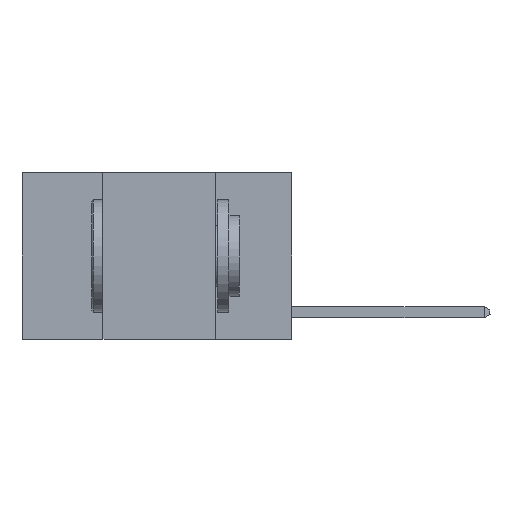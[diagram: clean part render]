
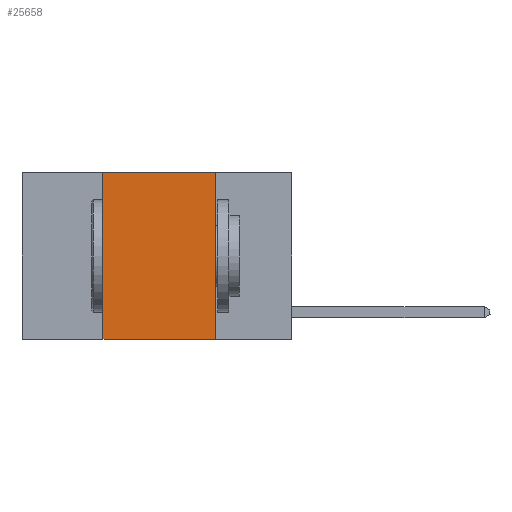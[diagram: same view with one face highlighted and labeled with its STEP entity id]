
A CAD part, left-side view. The second image highlights one B-rep face of the part: STEP entity #25658.
In plain terms, the highlighted planar face has unit normal (-1, 0, 0).
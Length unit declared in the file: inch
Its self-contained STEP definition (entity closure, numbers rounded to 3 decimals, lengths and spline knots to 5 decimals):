
#1001 = LINE ( 'NONE', #17578, #5790 ) ;
#1190 = CARTESIAN_POINT ( 'NONE',  ( 0., 0.17, 0. ) ) ;
#1494 = CARTESIAN_POINT ( 'NONE',  ( 0., 0.6, 0. ) ) ;
#2863 = CARTESIAN_POINT ( 'NONE',  ( 0., 0.42, 0. ) ) ;
#3183 = DIRECTION ( 'NONE',  ( 0., 0., -1. ) ) ;
#5790 = VECTOR ( 'NONE', #3183, 39.37008 ) ;
#6125 = EDGE_CURVE ( 'NONE', #17420, #9714, #18309, .T. ) ;
#6989 = VECTOR ( 'NONE', #9753, 39.37008 ) ;
#8087 = EDGE_CURVE ( 'NONE', #8499, #12565, #1001, .T. ) ;
#8123 = EDGE_LOOP ( 'NONE', ( #20190, #22357, #23123, #20723 ) ) ;
#8499 = VERTEX_POINT ( 'NONE', #1190 ) ;
#8555 = AXIS2_PLACEMENT_3D ( 'NONE', #1494, #11270, #13761 ) ;
#9714 = VERTEX_POINT ( 'NONE', #2863 ) ;
#9753 = DIRECTION ( 'NONE',  ( 0., 0., 1. ) ) ;
#11270 = DIRECTION ( 'NONE',  ( 1., 0., 0. ) ) ;
#11630 = EDGE_CURVE ( 'NONE', #9714, #8499, #18052, .T. ) ;
#12565 = VERTEX_POINT ( 'NONE', #26337 ) ;
#13349 = FACE_OUTER_BOUND ( 'NONE', #8123, .T. ) ;
#13761 = DIRECTION ( 'NONE',  ( 0., 0., -1. ) ) ;
#15602 = CARTESIAN_POINT ( 'NONE',  ( 0., 0.6, 0. ) ) ;
#16021 = DIRECTION ( 'NONE',  ( 0., -1., 0. ) ) ;
#17420 = VERTEX_POINT ( 'NONE', #19588 ) ;
#17578 = CARTESIAN_POINT ( 'NONE',  ( 0., 0.17, 0. ) ) ;
#17684 = LINE ( 'NONE', #25957, #22269 ) ;
#18052 = LINE ( 'NONE', #15602, #26066 ) ;
#18309 = LINE ( 'NONE', #20241, #6989 ) ;
#19588 = CARTESIAN_POINT ( 'NONE',  ( 0., 0.42, -0.37 ) ) ;
#19997 = PLANE ( 'NONE',  #8555 ) ;
#20148 = DIRECTION ( 'NONE',  ( 0., -1., 0. ) ) ;
#20190 = ORIENTED_EDGE ( 'NONE', *, *, #8087, .F. ) ;
#20241 = CARTESIAN_POINT ( 'NONE',  ( 0., 0.42, 0. ) ) ;
#20723 = ORIENTED_EDGE ( 'NONE', *, *, #23921, .T. ) ;
#22269 = VECTOR ( 'NONE', #20148, 39.37008 ) ;
#22357 = ORIENTED_EDGE ( 'NONE', *, *, #11630, .F. ) ;
#23123 = ORIENTED_EDGE ( 'NONE', *, *, #6125, .F. ) ;
#23921 = EDGE_CURVE ( 'NONE', #17420, #12565, #17684, .T. ) ;
#25658 = ADVANCED_FACE ( 'NONE', ( #13349 ), #19997, .F. ) ;
#25957 = CARTESIAN_POINT ( 'NONE',  ( 0., 0.6, -0.37 ) ) ;
#26066 = VECTOR ( 'NONE', #16021, 39.37008 ) ;
#26337 = CARTESIAN_POINT ( 'NONE',  ( 0., 0.17, -0.37 ) ) ;
